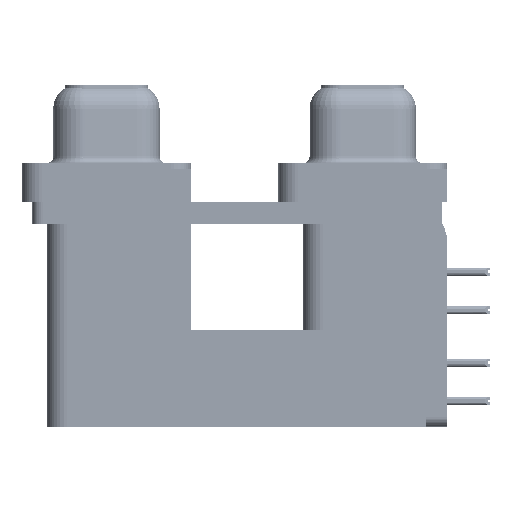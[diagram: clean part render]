
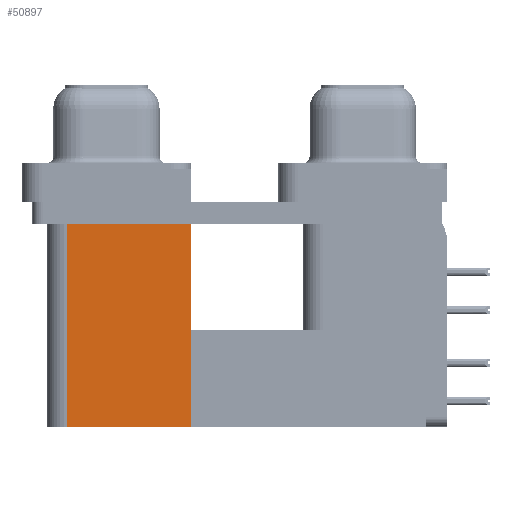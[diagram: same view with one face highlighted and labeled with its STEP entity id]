
A CAD part, left-side view. The second image highlights one B-rep face of the part: STEP entity #50897.
In plain terms, the highlighted planar face has unit normal (-1, 0, 0).
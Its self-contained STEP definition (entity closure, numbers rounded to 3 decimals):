
#1557 = CARTESIAN_POINT ( 'NONE',  ( 3.79, 12.775, -2.5 ) ) ;
#2888 = AXIS2_PLACEMENT_3D ( 'NONE', #16247, #45215, #45952 ) ;
#5876 = EDGE_CURVE ( 'NONE', #41443, #65288, #34260, .T. ) ;
#9040 = EDGE_CURVE ( 'NONE', #41443, #53935, #29734, .T. ) ;
#9819 = CARTESIAN_POINT ( 'NONE',  ( 3.79, 12.775, -19.2 ) ) ;
#14342 = EDGE_CURVE ( 'NONE', #53935, #58402, #30147, .T. ) ;
#16247 = CARTESIAN_POINT ( 'NONE',  ( 3.79, 12.775, -19.2 ) ) ;
#19686 = ORIENTED_EDGE ( 'NONE', *, *, #5876, .F. ) ;
#20879 = ORIENTED_EDGE ( 'NONE', *, *, #14342, .T. ) ;
#21890 = LINE ( 'NONE', #67458, #49754 ) ;
#23000 = PLANE ( 'NONE',  #2888 ) ;
#27160 = FACE_OUTER_BOUND ( 'NONE', #49712, .T. ) ;
#29734 = LINE ( 'NONE', #35780, #49935 ) ;
#30147 = LINE ( 'NONE', #1557, #46308 ) ;
#34260 = LINE ( 'NONE', #9819, #69894 ) ;
#35780 = CARTESIAN_POINT ( 'NONE',  ( 3.79, 12.775, -19.2 ) ) ;
#41102 = CARTESIAN_POINT ( 'NONE',  ( 3.79, 12.775, -2.5 ) ) ;
#41443 = VERTEX_POINT ( 'NONE', #67728 ) ;
#44829 = DIRECTION ( 'NONE',  ( 0., 0., 1. ) ) ;
#45215 = DIRECTION ( 'NONE',  ( 1., 0., 0. ) ) ;
#45952 = DIRECTION ( 'NONE',  ( 0., 0., -1. ) ) ;
#46308 = VECTOR ( 'NONE', #58447, 1000. ) ;
#49712 = EDGE_LOOP ( 'NONE', ( #20879, #64274, #19686, #61888 ) ) ;
#49754 = VECTOR ( 'NONE', #44829, 1000. ) ;
#49935 = VECTOR ( 'NONE', #59120, 1000. ) ;
#50897 = ADVANCED_FACE ( 'NONE', ( #27160 ), #23000, .F. ) ;
#50929 = EDGE_CURVE ( 'NONE', #65288, #58402, #21890, .T. ) ;
#53638 = CARTESIAN_POINT ( 'NONE',  ( 3.79, 21.975, -19.2 ) ) ;
#53935 = VERTEX_POINT ( 'NONE', #41102 ) ;
#58402 = VERTEX_POINT ( 'NONE', #71899 ) ;
#58447 = DIRECTION ( 'NONE',  ( 0., 1., 0. ) ) ;
#59120 = DIRECTION ( 'NONE',  ( 0., 0., 1. ) ) ;
#61888 = ORIENTED_EDGE ( 'NONE', *, *, #9040, .T. ) ;
#64274 = ORIENTED_EDGE ( 'NONE', *, *, #50929, .F. ) ;
#65288 = VERTEX_POINT ( 'NONE', #53638 ) ;
#67458 = CARTESIAN_POINT ( 'NONE',  ( 3.79, 21.975, -19.2 ) ) ;
#67728 = CARTESIAN_POINT ( 'NONE',  ( 3.79, 12.775, -19.2 ) ) ;
#69894 = VECTOR ( 'NONE', #73468, 1000. ) ;
#71899 = CARTESIAN_POINT ( 'NONE',  ( 3.79, 21.975, -2.5 ) ) ;
#73468 = DIRECTION ( 'NONE',  ( 0., 1., 0. ) ) ;
